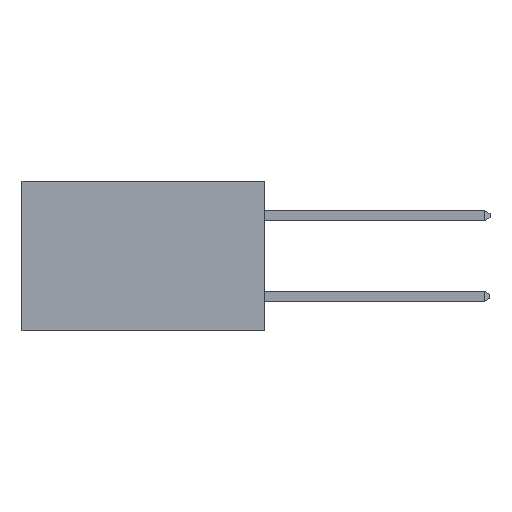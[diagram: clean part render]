
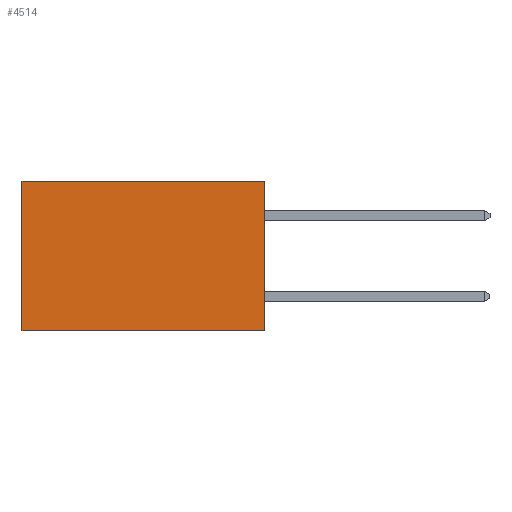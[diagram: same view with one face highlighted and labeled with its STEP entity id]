
A CAD part, left-side view. The second image highlights one B-rep face of the part: STEP entity #4514.
In plain terms, the highlighted planar face has unit normal (-1, 0, 0).
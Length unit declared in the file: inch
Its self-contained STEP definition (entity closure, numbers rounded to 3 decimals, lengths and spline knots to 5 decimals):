
#517 = DIRECTION ( 'NONE',  ( 0., 0., -1. ) ) ;
#974 = DIRECTION ( 'NONE',  ( 1., 0., 0. ) ) ;
#1181 = DIRECTION ( 'NONE',  ( 0., 1., 0. ) ) ;
#1792 = PLANE ( 'NONE',  #4159 ) ;
#1878 = EDGE_CURVE ( 'NONE', #4332, #2101, #10360, .T. ) ;
#1932 = EDGE_CURVE ( 'NONE', #4982, #4332, #6125, .T. ) ;
#2101 = VERTEX_POINT ( 'NONE', #4767 ) ;
#2775 = EDGE_LOOP ( 'NONE', ( #5024, #5154, #5801, #8512 ) ) ;
#2888 = FACE_OUTER_BOUND ( 'NONE', #2775, .T. ) ;
#3386 = EDGE_CURVE ( 'NONE', #8804, #2101, #8190, .T. ) ;
#3767 = VECTOR ( 'NONE', #1181, 39.37008 ) ;
#3921 = EDGE_CURVE ( 'NONE', #4982, #8804, #5713, .T. ) ;
#4159 = AXIS2_PLACEMENT_3D ( 'NONE', #5483, #974, #6778 ) ;
#4285 = DIRECTION ( 'NONE',  ( 0., 0., -1. ) ) ;
#4332 = VERTEX_POINT ( 'NONE', #5913 ) ;
#4514 = ADVANCED_FACE ( 'NONE', ( #2888 ), #1792, .F. ) ;
#4767 = CARTESIAN_POINT ( 'NONE',  ( 0.298, 0.6, -0.37 ) ) ;
#4982 = VERTEX_POINT ( 'NONE', #9022 ) ;
#5024 = ORIENTED_EDGE ( 'NONE', *, *, #1878, .T. ) ;
#5154 = ORIENTED_EDGE ( 'NONE', *, *, #3386, .F. ) ;
#5483 = CARTESIAN_POINT ( 'NONE',  ( 0.298, 0., 0. ) ) ;
#5713 = LINE ( 'NONE', #7590, #9604 ) ;
#5801 = ORIENTED_EDGE ( 'NONE', *, *, #3921, .F. ) ;
#5913 = CARTESIAN_POINT ( 'NONE',  ( 0.298, 0.6, 0. ) ) ;
#6125 = LINE ( 'NONE', #6347, #3767 ) ;
#6347 = CARTESIAN_POINT ( 'NONE',  ( 0.298, 0., 0. ) ) ;
#6511 = CARTESIAN_POINT ( 'NONE',  ( 0.298, 0.6, 0. ) ) ;
#6778 = DIRECTION ( 'NONE',  ( 0., 0., -1. ) ) ;
#7477 = DIRECTION ( 'NONE',  ( 0., 1., 0. ) ) ;
#7590 = CARTESIAN_POINT ( 'NONE',  ( 0.298, 0., 0. ) ) ;
#7913 = CARTESIAN_POINT ( 'NONE',  ( 0.298, 0., -0.37 ) ) ;
#8190 = LINE ( 'NONE', #7913, #10212 ) ;
#8376 = VECTOR ( 'NONE', #517, 39.37008 ) ;
#8512 = ORIENTED_EDGE ( 'NONE', *, *, #1932, .T. ) ;
#8804 = VERTEX_POINT ( 'NONE', #9088 ) ;
#9022 = CARTESIAN_POINT ( 'NONE',  ( 0.298, 0., 0. ) ) ;
#9088 = CARTESIAN_POINT ( 'NONE',  ( 0.298, 0., -0.37 ) ) ;
#9604 = VECTOR ( 'NONE', #4285, 39.37008 ) ;
#10212 = VECTOR ( 'NONE', #7477, 39.37008 ) ;
#10360 = LINE ( 'NONE', #6511, #8376 ) ;
